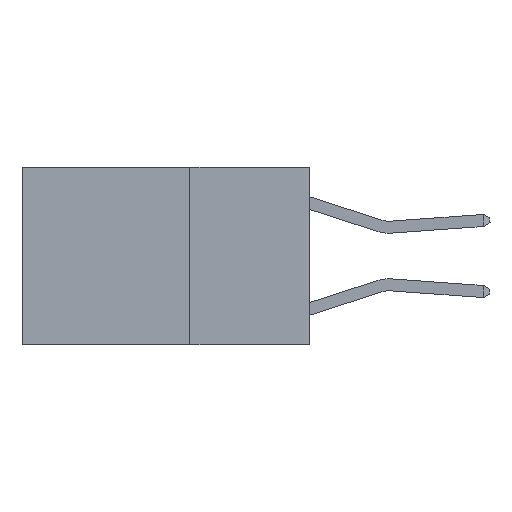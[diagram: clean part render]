
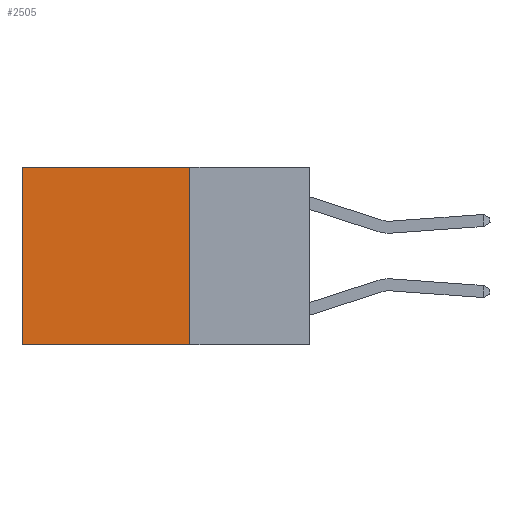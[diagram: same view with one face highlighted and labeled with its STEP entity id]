
A CAD part, left-side view. The second image highlights one B-rep face of the part: STEP entity #2505.
In plain terms, the highlighted planar face has unit normal (-1, 0, 0).
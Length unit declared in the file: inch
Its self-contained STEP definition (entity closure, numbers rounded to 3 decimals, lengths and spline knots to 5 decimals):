
#331 = DIRECTION ( 'NONE',  ( 1., 0., 0. ) ) ;
#683 = CARTESIAN_POINT ( 'NONE',  ( 0.2625, 0.25, 0. ) ) ;
#809 = DIRECTION ( 'NONE',  ( 0., 0., -1. ) ) ;
#1176 = VERTEX_POINT ( 'NONE', #10006 ) ;
#1594 = EDGE_LOOP ( 'NONE', ( #7847, #11981, #4322, #8291 ) ) ;
#2009 = DIRECTION ( 'NONE',  ( 0., 1., 0. ) ) ;
#2297 = FACE_OUTER_BOUND ( 'NONE', #1594, .T. ) ;
#2505 = ADVANCED_FACE ( 'NONE', ( #2297 ), #10563, .F. ) ;
#2756 = DIRECTION ( 'NONE',  ( 0., 1., 0. ) ) ;
#2853 = LINE ( 'NONE', #683, #11181 ) ;
#2864 = LINE ( 'NONE', #8033, #10538 ) ;
#3186 = VECTOR ( 'NONE', #2009, 39.37008 ) ;
#3986 = LINE ( 'NONE', #7125, #3186 ) ;
#4155 = VERTEX_POINT ( 'NONE', #7596 ) ;
#4322 = ORIENTED_EDGE ( 'NONE', *, *, #5185, .F. ) ;
#4476 = DIRECTION ( 'NONE',  ( 0., 0., -1. ) ) ;
#4663 = CARTESIAN_POINT ( 'NONE',  ( 0.2625, 0.25, 0. ) ) ;
#5185 = EDGE_CURVE ( 'NONE', #8146, #1176, #2853, .T. ) ;
#5656 = EDGE_CURVE ( 'NONE', #1176, #8682, #3986, .T. ) ;
#5911 = CARTESIAN_POINT ( 'NONE',  ( 0.2625, 0.25, 0. ) ) ;
#5948 = VECTOR ( 'NONE', #2756, 39.37008 ) ;
#7125 = CARTESIAN_POINT ( 'NONE',  ( 0.2625, 0.25, -0.37 ) ) ;
#7596 = CARTESIAN_POINT ( 'NONE',  ( 0.2625, 0.6, 0. ) ) ;
#7847 = ORIENTED_EDGE ( 'NONE', *, *, #8220, .T. ) ;
#8033 = CARTESIAN_POINT ( 'NONE',  ( 0.2625, 0.6, 0. ) ) ;
#8146 = VERTEX_POINT ( 'NONE', #5911 ) ;
#8220 = EDGE_CURVE ( 'NONE', #4155, #8682, #2864, .T. ) ;
#8291 = ORIENTED_EDGE ( 'NONE', *, *, #10439, .T. ) ;
#8682 = VERTEX_POINT ( 'NONE', #8892 ) ;
#8892 = CARTESIAN_POINT ( 'NONE',  ( 0.2625, 0.6, -0.37 ) ) ;
#9070 = LINE ( 'NONE', #4663, #5948 ) ;
#9118 = DIRECTION ( 'NONE',  ( 0., 0., -1. ) ) ;
#10006 = CARTESIAN_POINT ( 'NONE',  ( 0.2625, 0.25, -0.37 ) ) ;
#10439 = EDGE_CURVE ( 'NONE', #8146, #4155, #9070, .T. ) ;
#10538 = VECTOR ( 'NONE', #9118, 39.37008 ) ;
#10563 = PLANE ( 'NONE',  #13205 ) ;
#11181 = VECTOR ( 'NONE', #809, 39.37008 ) ;
#11813 = CARTESIAN_POINT ( 'NONE',  ( 0.2625, 0.25, 0. ) ) ;
#11981 = ORIENTED_EDGE ( 'NONE', *, *, #5656, .F. ) ;
#13205 = AXIS2_PLACEMENT_3D ( 'NONE', #11813, #331, #4476 ) ;
